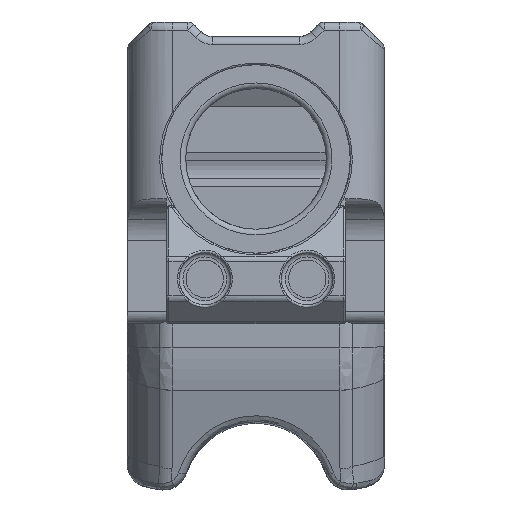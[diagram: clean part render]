
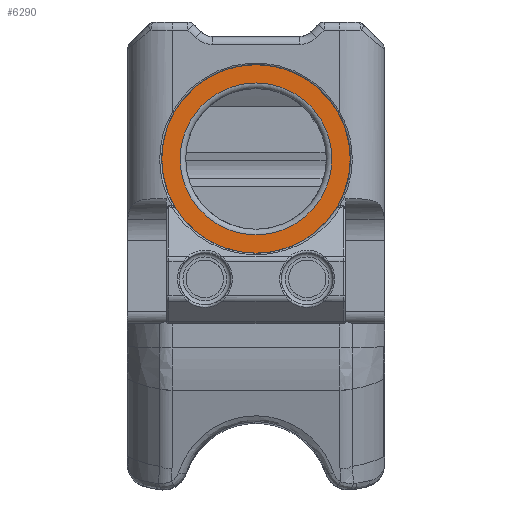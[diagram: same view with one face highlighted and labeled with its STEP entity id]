
A CAD part, front view. The second image highlights one B-rep face of the part: STEP entity #6290.
In plain terms, the highlighted planar face has unit normal (0, -1, 0).
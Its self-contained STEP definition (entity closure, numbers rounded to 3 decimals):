
#56=FACE_BOUND('',#1570,.T.);
#164=PLANE('',#6709);
#1171=FACE_OUTER_BOUND('',#1569,.T.);
#1569=EDGE_LOOP('',(#4225));
#1570=EDGE_LOOP('',(#4226));
#1986=CIRCLE('',#6708,9.425);
#1987=CIRCLE('',#6710,11.697);
#2566=VERTEX_POINT('',#9794);
#2567=VERTEX_POINT('',#9798);
#3192=EDGE_CURVE('',#2566,#2566,#1986,.T.);
#3193=EDGE_CURVE('',#2567,#2567,#1987,.T.);
#4225=ORIENTED_EDGE('',*,*,#3193,.T.);
#4226=ORIENTED_EDGE('',*,*,#3192,.F.);
#6290=ADVANCED_FACE('',(#1171,#56),#164,.T.);
#6708=AXIS2_PLACEMENT_3D('',#9796,#7462,#7463);
#6709=AXIS2_PLACEMENT_3D('',#9797,#7464,#7465);
#6710=AXIS2_PLACEMENT_3D('',#9799,#7466,#7467);
#7462=DIRECTION('center_axis',(0.,-1.,0.));
#7463=DIRECTION('ref_axis',(0.922,0.,0.388));
#7464=DIRECTION('center_axis',(0.,-1.,0.));
#7465=DIRECTION('ref_axis',(1.,0.,0.));
#7466=DIRECTION('center_axis',(0.,-1.,0.));
#7467=DIRECTION('ref_axis',(1.,0.,0.));
#9794=CARTESIAN_POINT('',(15.977,-18.733,-106.691));
#9796=CARTESIAN_POINT('Origin',(15.977,-18.733,-116.116));
#9797=CARTESIAN_POINT('Origin',(15.977,-18.733,-116.116));
#9798=CARTESIAN_POINT('',(15.977,-18.733,-127.813));
#9799=CARTESIAN_POINT('Origin',(15.977,-18.733,-116.116));
